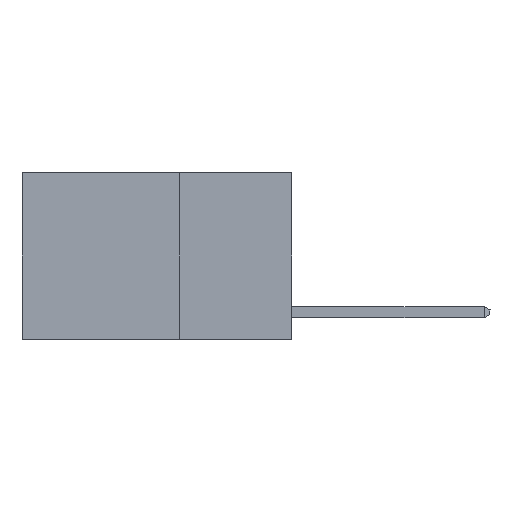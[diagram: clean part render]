
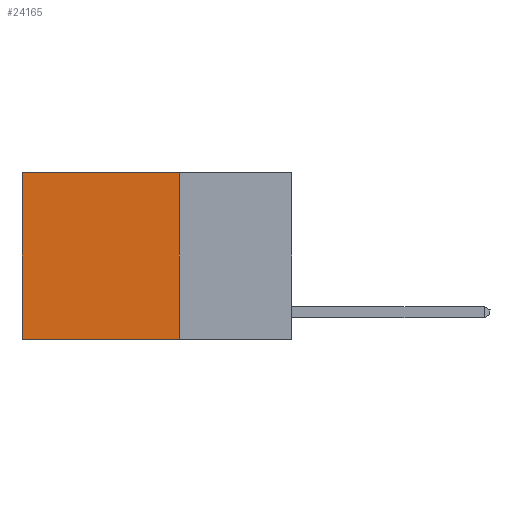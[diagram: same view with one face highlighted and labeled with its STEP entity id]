
A CAD part, left-side view. The second image highlights one B-rep face of the part: STEP entity #24165.
In plain terms, the highlighted planar face has unit normal (-1, 0, 0).
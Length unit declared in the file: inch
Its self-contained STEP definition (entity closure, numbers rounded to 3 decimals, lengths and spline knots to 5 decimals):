
#3207 = VECTOR ( 'NONE', #16860, 39.37008 ) ;
#4150 = VERTEX_POINT ( 'NONE', #18088 ) ;
#4193 = DIRECTION ( 'NONE',  ( 1., 0., 0. ) ) ;
#4917 = VERTEX_POINT ( 'NONE', #7875 ) ;
#5446 = CARTESIAN_POINT ( 'NONE',  ( 0.2625, 0.25, 0. ) ) ;
#7131 = VERTEX_POINT ( 'NONE', #7325 ) ;
#7325 = CARTESIAN_POINT ( 'NONE',  ( 0.2625, 0.25, -0.37 ) ) ;
#7384 = DIRECTION ( 'NONE',  ( 0., 0., -1. ) ) ;
#7475 = CARTESIAN_POINT ( 'NONE',  ( 0.2625, 0.6, 0. ) ) ;
#7875 = CARTESIAN_POINT ( 'NONE',  ( 0.2625, 0.6, -0.37 ) ) ;
#8853 = EDGE_CURVE ( 'NONE', #4150, #4917, #12253, .T. ) ;
#9869 = VECTOR ( 'NONE', #7384, 39.37008 ) ;
#10287 = EDGE_CURVE ( 'NONE', #7131, #4917, #12738, .T. ) ;
#10794 = VECTOR ( 'NONE', #21772, 39.37008 ) ;
#11311 = CARTESIAN_POINT ( 'NONE',  ( 0.2625, 0.25, 0. ) ) ;
#12253 = LINE ( 'NONE', #7475, #3207 ) ;
#12399 = LINE ( 'NONE', #5446, #10794 ) ;
#12738 = LINE ( 'NONE', #21519, #30274 ) ;
#13543 = EDGE_LOOP ( 'NONE', ( #24592, #18581, #24739, #17179 ) ) ;
#14113 = AXIS2_PLACEMENT_3D ( 'NONE', #11311, #4193, #21150 ) ;
#14146 = LINE ( 'NONE', #21535, #9869 ) ;
#14574 = DIRECTION ( 'NONE',  ( 0., 1., 0. ) ) ;
#14613 = EDGE_CURVE ( 'NONE', #20991, #4150, #12399, .T. ) ;
#15956 = CARTESIAN_POINT ( 'NONE',  ( 0.2625, 0.25, 0. ) ) ;
#16860 = DIRECTION ( 'NONE',  ( 0., 0., -1. ) ) ;
#17179 = ORIENTED_EDGE ( 'NONE', *, *, #14613, .T. ) ;
#18088 = CARTESIAN_POINT ( 'NONE',  ( 0.2625, 0.6, 0. ) ) ;
#18531 = PLANE ( 'NONE',  #14113 ) ;
#18581 = ORIENTED_EDGE ( 'NONE', *, *, #10287, .F. ) ;
#20991 = VERTEX_POINT ( 'NONE', #15956 ) ;
#20994 = FACE_OUTER_BOUND ( 'NONE', #13543, .T. ) ;
#21150 = DIRECTION ( 'NONE',  ( 0., 0., -1. ) ) ;
#21519 = CARTESIAN_POINT ( 'NONE',  ( 0.2625, 0.25, -0.37 ) ) ;
#21535 = CARTESIAN_POINT ( 'NONE',  ( 0.2625, 0.25, 0. ) ) ;
#21772 = DIRECTION ( 'NONE',  ( 0., 1., 0. ) ) ;
#24165 = ADVANCED_FACE ( 'NONE', ( #20994 ), #18531, .F. ) ;
#24592 = ORIENTED_EDGE ( 'NONE', *, *, #8853, .T. ) ;
#24739 = ORIENTED_EDGE ( 'NONE', *, *, #27953, .F. ) ;
#27953 = EDGE_CURVE ( 'NONE', #20991, #7131, #14146, .T. ) ;
#30274 = VECTOR ( 'NONE', #14574, 39.37008 ) ;
